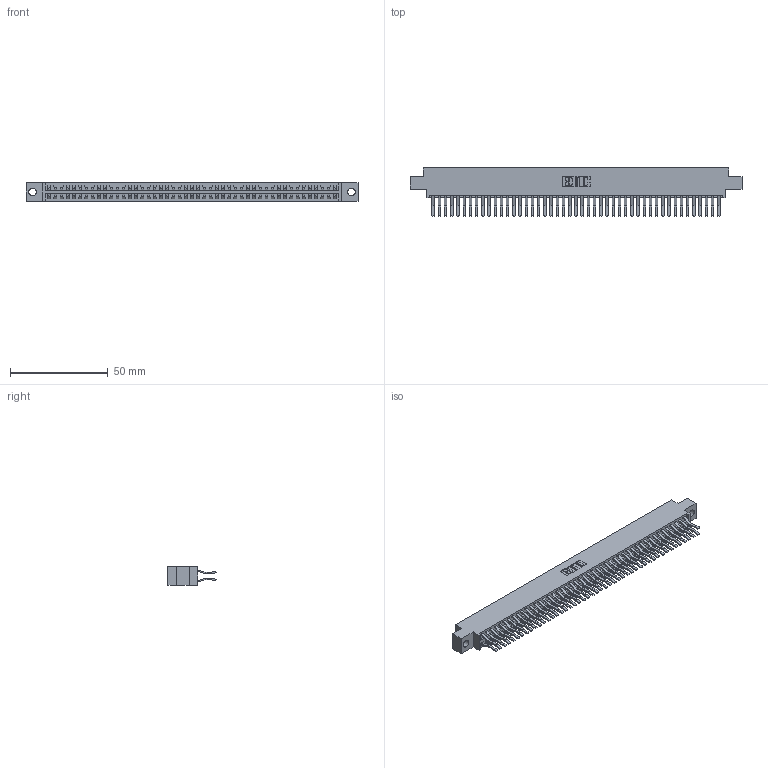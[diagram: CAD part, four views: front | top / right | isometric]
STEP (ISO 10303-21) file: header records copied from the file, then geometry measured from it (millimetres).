
FILE_DESCRIPTION (( 'STEP AP203' ), '1' );
FILE_NAME ('396-094-560-804.STEP', '2019-11-02T16:28:53', ( '' ), ( '' ), 'SwSTEP 2.0', 'SolidWorks 2016', '' );
FILE_SCHEMA (( 'CONFIG_CONTROL_DESIGN' ));
Length unit declared in the file: inch
Products named in the file (3): 345-292-001_560 Tail; 396-094-560-804; 346 Part_0.170 Offset - 0.156 Dia-TH
Assembly tree (95 placements, depth 2):
  396-094-560-804
    346 Part_0.170 Offset - 0.156 Dia-TH
    345-292-001_560 Tail  x94
Bounding box: 169.8 x 24.78 x 9.4 mm (x, y, z)
Volume: 16970 mm3; surface area: 25041.8 mm2
Topology: 95 solids, 95 shells, 5202 faces, 15475 edges, 10190 vertices
Faces by surface type: plane 3370, cylinder 1832
Entity records: 30223 total; most frequent: CARTESIAN_POINT 4976, ORIENTED_EDGE 4910, DIRECTION 4439, EDGE_CURVE 2455, LINE 2131, VECTOR 2131, VERTEX_POINT 1634, AXIS2_PLACEMENT_3D 1154
